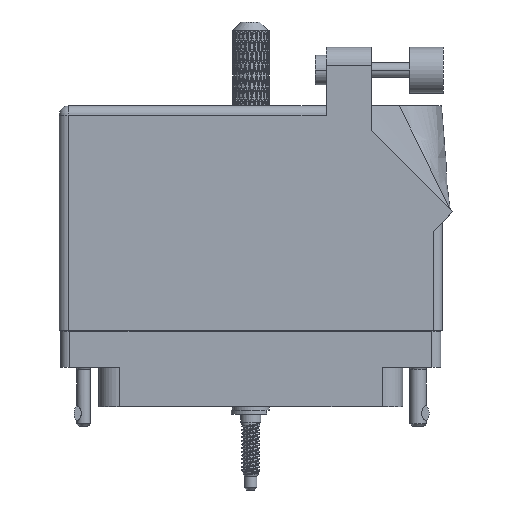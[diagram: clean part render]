
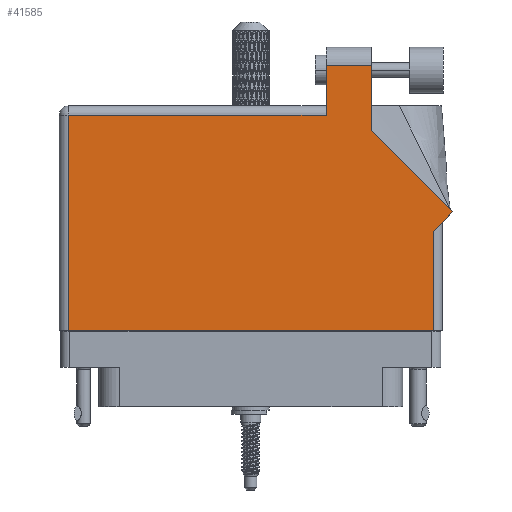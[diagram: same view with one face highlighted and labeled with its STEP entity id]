
A CAD part, front view. The second image highlights one B-rep face of the part: STEP entity #41585.
In plain terms, the highlighted face is planar.
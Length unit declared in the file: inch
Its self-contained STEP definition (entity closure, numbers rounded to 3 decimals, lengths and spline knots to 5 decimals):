
#715 = DIRECTION ( 'NONE',  ( 1., 0., 0. ) ) ;
#2839 = VECTOR ( 'NONE', #23296, 39.37008 ) ;
#4309 = CARTESIAN_POINT ( 'NONE',  ( 1.244, -0.1, 0.455 ) ) ;
#4528 = EDGE_CURVE ( 'NONE', #60713, #72305, #67232, .T. ) ;
#4796 = ORIENTED_EDGE ( 'NONE', *, *, #6536, .T. ) ;
#5062 = VECTOR ( 'NONE', #44605, 39.37008 ) ;
#6525 = CARTESIAN_POINT ( 'NONE',  ( 1.306, 0.637, 0.455 ) ) ;
#6536 = EDGE_CURVE ( 'NONE', #24923, #48437, #60995, .T. ) ;
#7281 = EDGE_CURVE ( 'NONE', #72305, #54305, #105244, .T. ) ;
#8050 = CARTESIAN_POINT ( 'NONE',  ( -1.306, 1.43, 0.455 ) ) ;
#8217 = CARTESIAN_POINT ( 'NONE',  ( -1.244, 1.368, 0.455 ) ) ;
#10011 = CARTESIAN_POINT ( 'NONE',  ( -1.244, -0.1, 0.455 ) ) ;
#10402 = ORIENTED_EDGE ( 'NONE', *, *, #100452, .T. ) ;
#11074 = LINE ( 'NONE', #21941, #101281 ) ;
#12262 = EDGE_CURVE ( 'NONE', #54305, #77339, #75072, .T. ) ;
#13820 = CARTESIAN_POINT ( 'NONE',  ( 0.82, 1.26442, 0.455 ) ) ;
#16637 = EDGE_CURVE ( 'NONE', #72980, #75814, #70138, .T. ) ;
#17424 = CARTESIAN_POINT ( 'NONE',  ( -1.306, 1.368, 0.455 ) ) ;
#18761 = DIRECTION ( 'NONE',  ( 0., -1., 0. ) ) ;
#20767 = ORIENTED_EDGE ( 'NONE', *, *, #114605, .T. ) ;
#21941 = CARTESIAN_POINT ( 'NONE',  ( 0.513, 1.43, 0.455 ) ) ;
#23175 = CARTESIAN_POINT ( 'NONE',  ( 1.244, 0.637, 0.455 ) ) ;
#23296 = DIRECTION ( 'NONE',  ( 0., 1., 0. ) ) ;
#24923 = VERTEX_POINT ( 'NONE', #56795 ) ;
#25301 = LINE ( 'NONE', #66260, #81507 ) ;
#27198 = CARTESIAN_POINT ( 'NONE',  ( 1.37671, 0.70771, 0.455 ) ) ;
#29891 = DIRECTION ( 'NONE',  ( -0.707, 0.707, 0. ) ) ;
#33187 = EDGE_CURVE ( 'NONE', #48437, #60713, #11074, .T. ) ;
#37296 = CARTESIAN_POINT ( 'NONE',  ( -1.244, -0.1, 0.455 ) ) ;
#37870 = CARTESIAN_POINT ( 'NONE',  ( -1.306, -0.1, 0.455 ) ) ;
#41585 = ADVANCED_FACE ( 'NONE', ( #117028 ), #45587, .F. ) ;
#43135 = VECTOR ( 'NONE', #109630, 39.37008 ) ;
#43804 = CARTESIAN_POINT ( 'NONE',  ( 0.82, 1.26442, 0.455 ) ) ;
#44605 = DIRECTION ( 'NONE',  ( -1., 0., 0. ) ) ;
#45587 = PLANE ( 'NONE',  #60255 ) ;
#48437 = VERTEX_POINT ( 'NONE', #105169 ) ;
#51219 = DIRECTION ( 'NONE',  ( 0., 0., -1. ) ) ;
#51616 = VECTOR ( 'NONE', #88906, 39.37008 ) ;
#54305 = VERTEX_POINT ( 'NONE', #10011 ) ;
#56795 = CARTESIAN_POINT ( 'NONE',  ( 0.82, 1.705, 0.455 ) ) ;
#58900 = ORIENTED_EDGE ( 'NONE', *, *, #16637, .T. ) ;
#60255 = AXIS2_PLACEMENT_3D ( 'NONE', #8050, #51219, #110639 ) ;
#60521 = LINE ( 'NONE', #13820, #2839 ) ;
#60713 = VERTEX_POINT ( 'NONE', #84002 ) ;
#60995 = LINE ( 'NONE', #100631, #43135 ) ;
#65054 = VERTEX_POINT ( 'NONE', #43804 ) ;
#66260 = CARTESIAN_POINT ( 'NONE',  ( 1.37671, 0.70771, 0.455 ) ) ;
#67232 = LINE ( 'NONE', #17424, #5062 ) ;
#70138 = LINE ( 'NONE', #6525, #110008 ) ;
#70303 = ORIENTED_EDGE ( 'NONE', *, *, #116348, .T. ) ;
#71237 = ORIENTED_EDGE ( 'NONE', *, *, #33187, .T. ) ;
#72087 = ORIENTED_EDGE ( 'NONE', *, *, #7281, .T. ) ;
#72305 = VERTEX_POINT ( 'NONE', #8217 ) ;
#72439 = CARTESIAN_POINT ( 'NONE',  ( 1.244, 0.575, 0.455 ) ) ;
#72980 = VERTEX_POINT ( 'NONE', #72439 ) ;
#75072 = LINE ( 'NONE', #37870, #86989 ) ;
#75689 = EDGE_LOOP ( 'NONE', ( #20767, #4796, #71237, #117244, #72087, #88507, #70303, #58900, #10402 ) ) ;
#75814 = VERTEX_POINT ( 'NONE', #27198 ) ;
#77339 = VERTEX_POINT ( 'NONE', #4309 ) ;
#80180 = VECTOR ( 'NONE', #18761, 39.37008 ) ;
#81507 = VECTOR ( 'NONE', #29891, 39.37008 ) ;
#84002 = CARTESIAN_POINT ( 'NONE',  ( 0.513, 1.368, 0.455 ) ) ;
#86989 = VECTOR ( 'NONE', #715, 39.37008 ) ;
#88507 = ORIENTED_EDGE ( 'NONE', *, *, #12262, .T. ) ;
#88906 = DIRECTION ( 'NONE',  ( 0., 1., 0. ) ) ;
#96711 = DIRECTION ( 'NONE',  ( 0., -1., 0. ) ) ;
#100452 = EDGE_CURVE ( 'NONE', #75814, #65054, #25301, .T. ) ;
#100631 = CARTESIAN_POINT ( 'NONE',  ( 0.513, 1.705, 0.455 ) ) ;
#101281 = VECTOR ( 'NONE', #96711, 39.37008 ) ;
#105169 = CARTESIAN_POINT ( 'NONE',  ( 0.513, 1.705, 0.455 ) ) ;
#105244 = LINE ( 'NONE', #37296, #80180 ) ;
#109630 = DIRECTION ( 'NONE',  ( -1., 0., 0. ) ) ;
#110008 = VECTOR ( 'NONE', #112257, 39.37008 ) ;
#110639 = DIRECTION ( 'NONE',  ( -1., 0., 0. ) ) ;
#112257 = DIRECTION ( 'NONE',  ( 0.707, 0.707, 0. ) ) ;
#114605 = EDGE_CURVE ( 'NONE', #65054, #24923, #60521, .T. ) ;
#116348 = EDGE_CURVE ( 'NONE', #77339, #72980, #116537, .T. ) ;
#116537 = LINE ( 'NONE', #23175, #51616 ) ;
#117028 = FACE_OUTER_BOUND ( 'NONE', #75689, .T. ) ;
#117244 = ORIENTED_EDGE ( 'NONE', *, *, #4528, .T. ) ;
